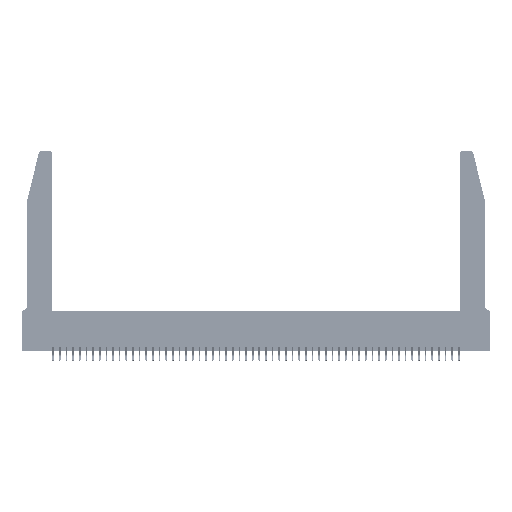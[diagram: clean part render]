
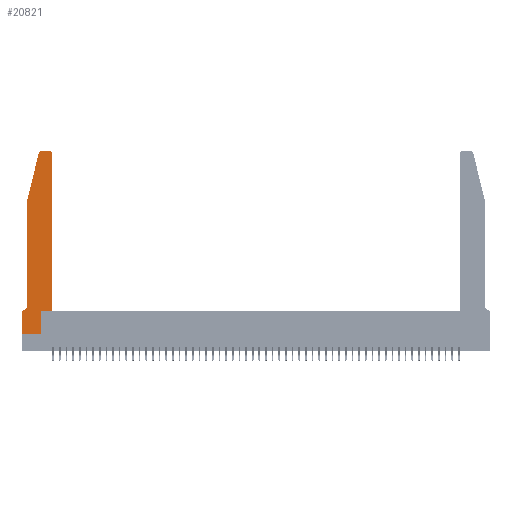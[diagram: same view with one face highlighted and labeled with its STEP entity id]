
A CAD part, top view. The second image highlights one B-rep face of the part: STEP entity #20821.
In plain terms, the highlighted planar face has unit normal (0, 0, 1).
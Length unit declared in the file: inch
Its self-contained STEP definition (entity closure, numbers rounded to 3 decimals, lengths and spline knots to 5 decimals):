
#61 = ORIENTED_EDGE ( 'NONE', *, *, #47972, .T. ) ;
#149 = ORIENTED_EDGE ( 'NONE', *, *, #44510, .T. ) ;
#185 = CARTESIAN_POINT ( 'NONE',  ( 0., 0., 0.37 ) ) ;
#682 = AXIS2_PLACEMENT_3D ( 'NONE', #9972, #37641, #13995 ) ;
#705 = ORIENTED_EDGE ( 'NONE', *, *, #3175, .T. ) ;
#1965 = CARTESIAN_POINT ( 'NONE',  ( 0.2865, 0., 0.37 ) ) ;
#2021 = ORIENTED_EDGE ( 'NONE', *, *, #47388, .T. ) ;
#2319 = DIRECTION ( 'NONE',  ( 0., 0., 1. ) ) ;
#2675 = LINE ( 'NONE', #46557, #23816 ) ;
#3175 = EDGE_CURVE ( 'NONE', #28012, #30635, #44416, .T. ) ;
#3353 = CARTESIAN_POINT ( 'NONE',  ( 0., 0., 0.37 ) ) ;
#3412 = VERTEX_POINT ( 'NONE', #3974 ) ;
#3974 = CARTESIAN_POINT ( 'NONE',  ( 0.4505, 2.72, 0.37 ) ) ;
#4116 = DIRECTION ( 'NONE',  ( 0., -1., 0. ) ) ;
#4729 = VECTOR ( 'NONE', #15791, 39.37008 ) ;
#5432 = EDGE_CURVE ( 'NONE', #30635, #31099, #41161, .T. ) ;
#5588 = VERTEX_POINT ( 'NONE', #1965 ) ;
#6877 = ORIENTED_EDGE ( 'NONE', *, *, #15045, .T. ) ;
#7060 = VERTEX_POINT ( 'NONE', #14816 ) ;
#7206 = CARTESIAN_POINT ( 'NONE',  ( 0.25487, 2.72718, 0.37 ) ) ;
#7323 = DIRECTION ( 'NONE',  ( 1., 0., 0. ) ) ;
#7383 = DIRECTION ( 'NONE',  ( 0., 1., 0. ) ) ;
#7711 = EDGE_CURVE ( 'NONE', #42854, #27507, #2675, .T. ) ;
#7919 = LINE ( 'NONE', #3353, #48549 ) ;
#8813 = VERTEX_POINT ( 'NONE', #19031 ) ;
#9112 = VERTEX_POINT ( 'NONE', #44210 ) ;
#9456 = DIRECTION ( 'NONE',  ( 0., 1., 0. ) ) ;
#9502 = CARTESIAN_POINT ( 'NONE',  ( 0.2865, 0.35, 0.37 ) ) ;
#9972 = CARTESIAN_POINT ( 'NONE',  ( 0.0055, 0.42, 0.37 ) ) ;
#9989 = ORIENTED_EDGE ( 'NONE', *, *, #39082, .T. ) ;
#10083 = CARTESIAN_POINT ( 'NONE',  ( 0.0755, 2., 0.37 ) ) ;
#11519 = VERTEX_POINT ( 'NONE', #9502 ) ;
#13995 = DIRECTION ( 'NONE',  ( -1., 0., 0. ) ) ;
#14258 = EDGE_CURVE ( 'NONE', #8813, #5588, #7919, .T. ) ;
#14389 = ORIENTED_EDGE ( 'NONE', *, *, #46520, .T. ) ;
#14816 = CARTESIAN_POINT ( 'NONE',  ( 0.4505, 0.35, 0.37 ) ) ;
#15045 = EDGE_CURVE ( 'NONE', #9112, #49568, #35078, .T. ) ;
#15214 = CARTESIAN_POINT ( 'NONE',  ( 0.4505, 0.35, 0.37 ) ) ;
#15791 = DIRECTION ( 'NONE',  ( -1., 0., 0. ) ) ;
#15904 = CIRCLE ( 'NONE', #22690, 0.03 ) ;
#16229 = ORIENTED_EDGE ( 'NONE', *, *, #24795, .T. ) ;
#17596 = DIRECTION ( 'NONE',  ( 1., 0., 0. ) ) ;
#19031 = CARTESIAN_POINT ( 'NONE',  ( 0., 0., 0.37 ) ) ;
#19064 = VECTOR ( 'NONE', #36543, 39.37008 ) ;
#20301 = CARTESIAN_POINT ( 'NONE',  ( 0.4205, 2.75, 0.37 ) ) ;
#20821 = ADVANCED_FACE ( 'NONE', ( #36929 ), #44880, .T. ) ;
#20887 = CARTESIAN_POINT ( 'NONE',  ( 0.0755, 2., 0.37 ) ) ;
#21245 = ORIENTED_EDGE ( 'NONE', *, *, #47433, .T. ) ;
#21501 = CARTESIAN_POINT ( 'NONE',  ( 0.2865, 0.35, 0.37 ) ) ;
#21559 = CARTESIAN_POINT ( 'NONE',  ( 0.0755, 0.42, 0.37 ) ) ;
#21825 = ORIENTED_EDGE ( 'NONE', *, *, #5432, .T. ) ;
#22508 = DIRECTION ( 'NONE',  ( 0., 0., 1. ) ) ;
#22690 = AXIS2_PLACEMENT_3D ( 'NONE', #26085, #2319, #30004 ) ;
#23678 = LINE ( 'NONE', #38617, #43259 ) ;
#23816 = VECTOR ( 'NONE', #50456, 39.37008 ) ;
#24066 = EDGE_LOOP ( 'NONE', ( #30406, #61, #705, #21825, #16229, #6877, #9989, #31097, #149, #21245, #14389, #2021 ) ) ;
#24249 = CARTESIAN_POINT ( 'NONE',  ( 0., 0.35, 0.37 ) ) ;
#24658 = CARTESIAN_POINT ( 'NONE',  ( 0.284, 2.75, 0.37 ) ) ;
#24795 = EDGE_CURVE ( 'NONE', #31099, #9112, #42970, .T. ) ;
#24997 = VECTOR ( 'NONE', #7383, 39.37008 ) ;
#26085 = CARTESIAN_POINT ( 'NONE',  ( 0.284, 2.72, 0.37 ) ) ;
#27507 = VERTEX_POINT ( 'NONE', #24658 ) ;
#28012 = VERTEX_POINT ( 'NONE', #7206 ) ;
#30004 = DIRECTION ( 'NONE',  ( 1., 0., 0. ) ) ;
#30406 = ORIENTED_EDGE ( 'NONE', *, *, #7711, .T. ) ;
#30635 = VERTEX_POINT ( 'NONE', #10083 ) ;
#31097 = ORIENTED_EDGE ( 'NONE', *, *, #14258, .T. ) ;
#31099 = VERTEX_POINT ( 'NONE', #21559 ) ;
#32529 = AXIS2_PLACEMENT_3D ( 'NONE', #45947, #22508, #49836 ) ;
#32880 = VECTOR ( 'NONE', #4116, 39.37008 ) ;
#34044 = VECTOR ( 'NONE', #34275, 39.37008 ) ;
#34275 = DIRECTION ( 'NONE',  ( -0.239, -0.971, 0. ) ) ;
#35078 = LINE ( 'NONE', #47193, #4729 ) ;
#35448 = LINE ( 'NONE', #15214, #24997 ) ;
#36543 = DIRECTION ( 'NONE',  ( 0., -1., 0. ) ) ;
#36572 = CIRCLE ( 'NONE', #32529, 0.03 ) ;
#36929 = FACE_OUTER_BOUND ( 'NONE', #24066, .T. ) ;
#37221 = CARTESIAN_POINT ( 'NONE',  ( 0., 0.35, 0.37 ) ) ;
#37641 = DIRECTION ( 'NONE',  ( 0., 0., -1. ) ) ;
#38617 = CARTESIAN_POINT ( 'NONE',  ( 0.4505, 0.35, 0.37 ) ) ;
#39082 = EDGE_CURVE ( 'NONE', #49568, #8813, #44488, .T. ) ;
#41109 = DIRECTION ( 'NONE',  ( 0., 0., 1. ) ) ;
#41161 = LINE ( 'NONE', #20887, #19064 ) ;
#42532 = DIRECTION ( 'NONE',  ( 1., 0., 0. ) ) ;
#42854 = VERTEX_POINT ( 'NONE', #20301 ) ;
#42970 = CIRCLE ( 'NONE', #682, 0.07 ) ;
#43259 = VECTOR ( 'NONE', #42532, 39.37008 ) ;
#43484 = VECTOR ( 'NONE', #9456, 39.37008 ) ;
#44210 = CARTESIAN_POINT ( 'NONE',  ( 0.0055, 0.35, 0.37 ) ) ;
#44416 = LINE ( 'NONE', #45872, #34044 ) ;
#44488 = LINE ( 'NONE', #185, #32880 ) ;
#44510 = EDGE_CURVE ( 'NONE', #5588, #11519, #44703, .T. ) ;
#44703 = LINE ( 'NONE', #21501, #43484 ) ;
#44880 = PLANE ( 'NONE',  #49362 ) ;
#45872 = CARTESIAN_POINT ( 'NONE',  ( 0.0755, 2., 0.37 ) ) ;
#45947 = CARTESIAN_POINT ( 'NONE',  ( 0.4205, 2.72, 0.37 ) ) ;
#46520 = EDGE_CURVE ( 'NONE', #7060, #3412, #35448, .T. ) ;
#46557 = CARTESIAN_POINT ( 'NONE',  ( 0.2605, 2.75, 0.37 ) ) ;
#47193 = CARTESIAN_POINT ( 'NONE',  ( 0.0755, 0.35, 0.37 ) ) ;
#47388 = EDGE_CURVE ( 'NONE', #3412, #42854, #36572, .T. ) ;
#47433 = EDGE_CURVE ( 'NONE', #11519, #7060, #23678, .T. ) ;
#47972 = EDGE_CURVE ( 'NONE', #27507, #28012, #15904, .T. ) ;
#48549 = VECTOR ( 'NONE', #7323, 39.37008 ) ;
#49362 = AXIS2_PLACEMENT_3D ( 'NONE', #37221, #41109, #17596 ) ;
#49568 = VERTEX_POINT ( 'NONE', #24249 ) ;
#49836 = DIRECTION ( 'NONE',  ( 1., 0., 0. ) ) ;
#50456 = DIRECTION ( 'NONE',  ( -1., 0., 0. ) ) ;
